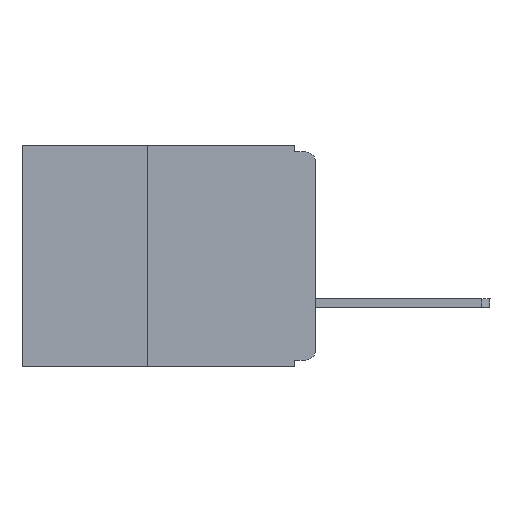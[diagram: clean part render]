
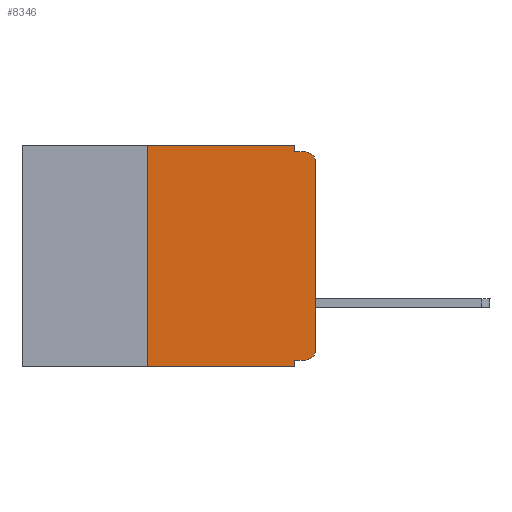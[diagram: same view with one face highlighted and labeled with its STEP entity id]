
A CAD part, left-side view. The second image highlights one B-rep face of the part: STEP entity #8346.
In plain terms, the highlighted planar face has unit normal (-1, 0, 0).
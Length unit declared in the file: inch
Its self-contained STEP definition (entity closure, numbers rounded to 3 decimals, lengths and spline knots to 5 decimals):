
#104 = DIRECTION ( 'NONE',  ( -1., 0., 0. ) ) ;
#352 = ORIENTED_EDGE ( 'NONE', *, *, #8799, .F. ) ;
#543 = ORIENTED_EDGE ( 'NONE', *, *, #10641, .F. ) ;
#574 = AXIS2_PLACEMENT_3D ( 'NONE', #11404, #104, #12434 ) ;
#696 = CARTESIAN_POINT ( 'NONE',  ( 0., 0., -0.01 ) ) ;
#832 = CARTESIAN_POINT ( 'NONE',  ( 0., 0.031, 0. ) ) ;
#1272 = EDGE_CURVE ( 'NONE', #10580, #5729, #8878, .T. ) ;
#1663 = CARTESIAN_POINT ( 'NONE',  ( 0., 0.25, -0.33 ) ) ;
#1979 = CARTESIAN_POINT ( 'NONE',  ( 0., 0., -0.32 ) ) ;
#1998 = LINE ( 'NONE', #2918, #3728 ) ;
#2112 = FACE_OUTER_BOUND ( 'NONE', #11439, .T. ) ;
#2472 = EDGE_CURVE ( 'NONE', #8184, #6476, #3647, .T. ) ;
#2518 = EDGE_CURVE ( 'NONE', #7907, #7186, #11718, .T. ) ;
#2918 = CARTESIAN_POINT ( 'NONE',  ( 0., 0.031, 0. ) ) ;
#2990 = LINE ( 'NONE', #1979, #10864 ) ;
#3056 = CARTESIAN_POINT ( 'NONE',  ( 0., 0.25, -0.33 ) ) ;
#3103 = CARTESIAN_POINT ( 'NONE',  ( 0., 0.437, 0. ) ) ;
#3115 = CARTESIAN_POINT ( 'NONE',  ( 0., 0.015, -0.025 ) ) ;
#3239 = ORIENTED_EDGE ( 'NONE', *, *, #8721, .F. ) ;
#3241 = ORIENTED_EDGE ( 'NONE', *, *, #4755, .F. ) ;
#3368 = ORIENTED_EDGE ( 'NONE', *, *, #2472, .T. ) ;
#3507 = CARTESIAN_POINT ( 'NONE',  ( 0., 0., -0.305 ) ) ;
#3647 = CIRCLE ( 'NONE', #11982, 0.015 ) ;
#3728 = VECTOR ( 'NONE', #9356, 39.37008 ) ;
#3952 = DIRECTION ( 'NONE',  ( 0., 0., -1. ) ) ;
#4120 = DIRECTION ( 'NONE',  ( -1., 0., 0. ) ) ;
#4311 = VECTOR ( 'NONE', #12934, 39.37008 ) ;
#4477 = LINE ( 'NONE', #1663, #11425 ) ;
#4556 = VERTEX_POINT ( 'NONE', #832 ) ;
#4755 = EDGE_CURVE ( 'NONE', #4556, #13279, #1998, .T. ) ;
#4853 = CARTESIAN_POINT ( 'NONE',  ( 0., 0.015, -0.01 ) ) ;
#4860 = DIRECTION ( 'NONE',  ( 0., 0., -1. ) ) ;
#4892 = CARTESIAN_POINT ( 'NONE',  ( 0., 0., -0.025 ) ) ;
#4901 = CARTESIAN_POINT ( 'NONE',  ( 0., 0., 0. ) ) ;
#5210 = LINE ( 'NONE', #3103, #13112 ) ;
#5729 = VERTEX_POINT ( 'NONE', #3507 ) ;
#6055 = AXIS2_PLACEMENT_3D ( 'NONE', #9203, #9165, #3952 ) ;
#6449 = VERTEX_POINT ( 'NONE', #8032 ) ;
#6476 = VERTEX_POINT ( 'NONE', #4853 ) ;
#7031 = CARTESIAN_POINT ( 'NONE',  ( 0., 0.031, -0.33 ) ) ;
#7186 = VERTEX_POINT ( 'NONE', #8513 ) ;
#7215 = ORIENTED_EDGE ( 'NONE', *, *, #1272, .T. ) ;
#7682 = VERTEX_POINT ( 'NONE', #10943 ) ;
#7907 = VERTEX_POINT ( 'NONE', #3056 ) ;
#8008 = LINE ( 'NONE', #4901, #9470 ) ;
#8032 = CARTESIAN_POINT ( 'NONE',  ( 0., 0.25, 0. ) ) ;
#8184 = VERTEX_POINT ( 'NONE', #4892 ) ;
#8195 = DIRECTION ( 'NONE',  ( 0., 0., -1. ) ) ;
#8346 = ADVANCED_FACE ( 'NONE', ( #2112 ), #10219, .F. ) ;
#8450 = ORIENTED_EDGE ( 'NONE', *, *, #13150, .T. ) ;
#8513 = CARTESIAN_POINT ( 'NONE',  ( 0., 0.031, -0.33 ) ) ;
#8615 = CARTESIAN_POINT ( 'NONE',  ( 0., 0.031, -0.01 ) ) ;
#8721 = EDGE_CURVE ( 'NONE', #7907, #6449, #4477, .T. ) ;
#8799 = EDGE_CURVE ( 'NONE', #13279, #6476, #9952, .T. ) ;
#8878 = CIRCLE ( 'NONE', #574, 0.015 ) ;
#8918 = ORIENTED_EDGE ( 'NONE', *, *, #11554, .F. ) ;
#9165 = DIRECTION ( 'NONE',  ( 1., 0., 0. ) ) ;
#9189 = DIRECTION ( 'NONE',  ( 0., 0., 1. ) ) ;
#9203 = CARTESIAN_POINT ( 'NONE',  ( 0., 0.437, 0. ) ) ;
#9356 = DIRECTION ( 'NONE',  ( 0., 0., -1. ) ) ;
#9470 = VECTOR ( 'NONE', #10226, 39.37008 ) ;
#9473 = VECTOR ( 'NONE', #9504, 39.37008 ) ;
#9504 = DIRECTION ( 'NONE',  ( 0., -1., 0. ) ) ;
#9952 = LINE ( 'NONE', #696, #4311 ) ;
#10219 = PLANE ( 'NONE',  #6055 ) ;
#10226 = DIRECTION ( 'NONE',  ( 0., 0., 1. ) ) ;
#10580 = VERTEX_POINT ( 'NONE', #12012 ) ;
#10641 = EDGE_CURVE ( 'NONE', #10580, #7682, #2990, .T. ) ;
#10864 = VECTOR ( 'NONE', #11335, 39.37008 ) ;
#10943 = CARTESIAN_POINT ( 'NONE',  ( 0., 0.031, -0.32 ) ) ;
#11147 = ORIENTED_EDGE ( 'NONE', *, *, #2518, .T. ) ;
#11335 = DIRECTION ( 'NONE',  ( 0., 1., 0. ) ) ;
#11404 = CARTESIAN_POINT ( 'NONE',  ( 0., 0.015, -0.305 ) ) ;
#11425 = VECTOR ( 'NONE', #9189, 39.37008 ) ;
#11433 = EDGE_CURVE ( 'NONE', #7682, #7186, #11515, .T. ) ;
#11439 = EDGE_LOOP ( 'NONE', ( #8450, #3368, #352, #3241, #8918, #3239, #11147, #12219, #543, #7215 ) ) ;
#11515 = LINE ( 'NONE', #7031, #11682 ) ;
#11554 = EDGE_CURVE ( 'NONE', #6449, #4556, #5210, .T. ) ;
#11682 = VECTOR ( 'NONE', #4860, 39.37008 ) ;
#11718 = LINE ( 'NONE', #12633, #9473 ) ;
#11982 = AXIS2_PLACEMENT_3D ( 'NONE', #3115, #4120, #8195 ) ;
#12012 = CARTESIAN_POINT ( 'NONE',  ( 0., 0.015, -0.32 ) ) ;
#12219 = ORIENTED_EDGE ( 'NONE', *, *, #11433, .F. ) ;
#12317 = DIRECTION ( 'NONE',  ( 0., -1., 0. ) ) ;
#12434 = DIRECTION ( 'NONE',  ( 0., 0., -1. ) ) ;
#12633 = CARTESIAN_POINT ( 'NONE',  ( 0., 0.437, -0.33 ) ) ;
#12934 = DIRECTION ( 'NONE',  ( 0., -1., 0. ) ) ;
#13112 = VECTOR ( 'NONE', #12317, 39.37008 ) ;
#13150 = EDGE_CURVE ( 'NONE', #5729, #8184, #8008, .T. ) ;
#13279 = VERTEX_POINT ( 'NONE', #8615 ) ;
